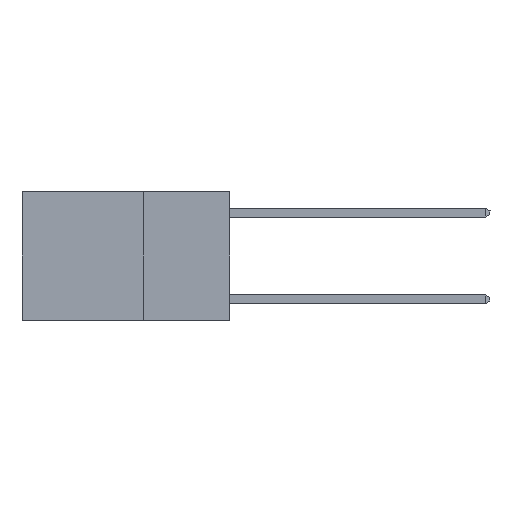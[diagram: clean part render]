
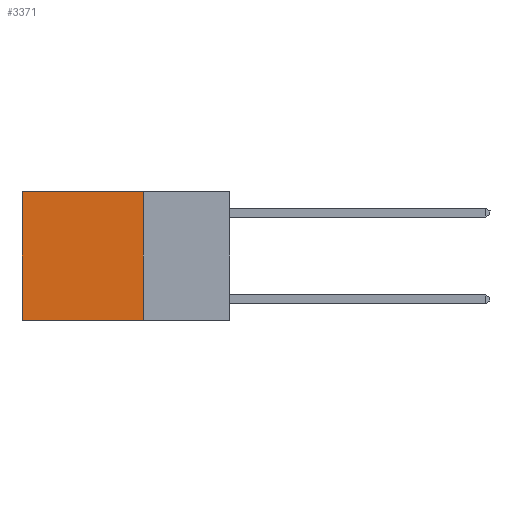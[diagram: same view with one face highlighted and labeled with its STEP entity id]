
A CAD part, left-side view. The second image highlights one B-rep face of the part: STEP entity #3371.
In plain terms, the highlighted planar face has unit normal (-1, 0, 0).
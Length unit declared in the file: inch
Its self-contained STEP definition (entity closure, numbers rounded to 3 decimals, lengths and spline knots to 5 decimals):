
#752 = VERTEX_POINT ( 'NONE', #20962 ) ;
#1059 = EDGE_CURVE ( 'NONE', #27113, #752, #25564, .T. ) ;
#1924 = AXIS2_PLACEMENT_3D ( 'NONE', #22381, #8945, #24626 ) ;
#2783 = DIRECTION ( 'NONE',  ( 0., 0., -1. ) ) ;
#3371 = ADVANCED_FACE ( 'NONE', ( #25417 ), #20144, .F. ) ;
#4026 = VERTEX_POINT ( 'NONE', #23168 ) ;
#4684 = ORIENTED_EDGE ( 'NONE', *, *, #1059, .F. ) ;
#4811 = CARTESIAN_POINT ( 'NONE',  ( 0.2625, 0.25, -0.37 ) ) ;
#7281 = CARTESIAN_POINT ( 'NONE',  ( 0.2625, 0.6, 0. ) ) ;
#7788 = LINE ( 'NONE', #7281, #27748 ) ;
#8487 = VERTEX_POINT ( 'NONE', #26518 ) ;
#8945 = DIRECTION ( 'NONE',  ( 1., 0., 0. ) ) ;
#9155 = EDGE_CURVE ( 'NONE', #4026, #752, #7788, .T. ) ;
#10348 = ORIENTED_EDGE ( 'NONE', *, *, #22088, .F. ) ;
#12571 = VECTOR ( 'NONE', #17369, 39.37008 ) ;
#12927 = LINE ( 'NONE', #19826, #19270 ) ;
#15864 = EDGE_LOOP ( 'NONE', ( #24018, #4684, #10348, #20926 ) ) ;
#16426 = LINE ( 'NONE', #24013, #12571 ) ;
#17369 = DIRECTION ( 'NONE',  ( 0., 0., -1. ) ) ;
#17457 = DIRECTION ( 'NONE',  ( 0., 1., 0. ) ) ;
#19270 = VECTOR ( 'NONE', #17457, 39.37008 ) ;
#19826 = CARTESIAN_POINT ( 'NONE',  ( 0.2625, 0.25, 0. ) ) ;
#20144 = PLANE ( 'NONE',  #1924 ) ;
#20926 = ORIENTED_EDGE ( 'NONE', *, *, #22135, .T. ) ;
#20962 = CARTESIAN_POINT ( 'NONE',  ( 0.2625, 0.6, -0.37 ) ) ;
#22088 = EDGE_CURVE ( 'NONE', #8487, #27113, #16426, .T. ) ;
#22135 = EDGE_CURVE ( 'NONE', #8487, #4026, #12927, .T. ) ;
#22381 = CARTESIAN_POINT ( 'NONE',  ( 0.2625, 0.25, 0. ) ) ;
#23168 = CARTESIAN_POINT ( 'NONE',  ( 0.2625, 0.6, 0. ) ) ;
#23596 = DIRECTION ( 'NONE',  ( 0., 1., 0. ) ) ;
#24013 = CARTESIAN_POINT ( 'NONE',  ( 0.2625, 0.25, 0. ) ) ;
#24018 = ORIENTED_EDGE ( 'NONE', *, *, #9155, .T. ) ;
#24626 = DIRECTION ( 'NONE',  ( 0., 0., -1. ) ) ;
#25417 = FACE_OUTER_BOUND ( 'NONE', #15864, .T. ) ;
#25564 = LINE ( 'NONE', #25659, #27663 ) ;
#25659 = CARTESIAN_POINT ( 'NONE',  ( 0.2625, 0.25, -0.37 ) ) ;
#26518 = CARTESIAN_POINT ( 'NONE',  ( 0.2625, 0.25, 0. ) ) ;
#27113 = VERTEX_POINT ( 'NONE', #4811 ) ;
#27663 = VECTOR ( 'NONE', #23596, 39.37008 ) ;
#27748 = VECTOR ( 'NONE', #2783, 39.37008 ) ;
